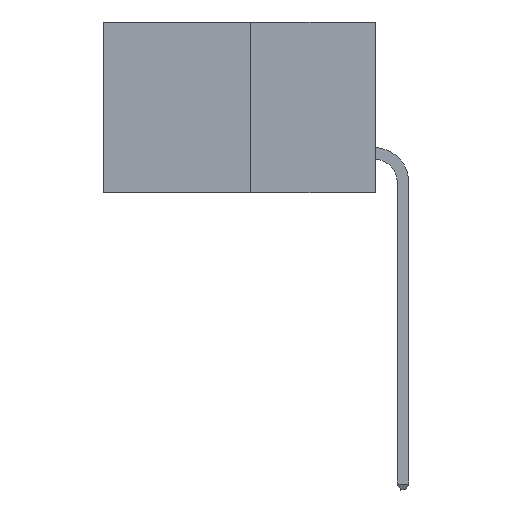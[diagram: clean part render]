
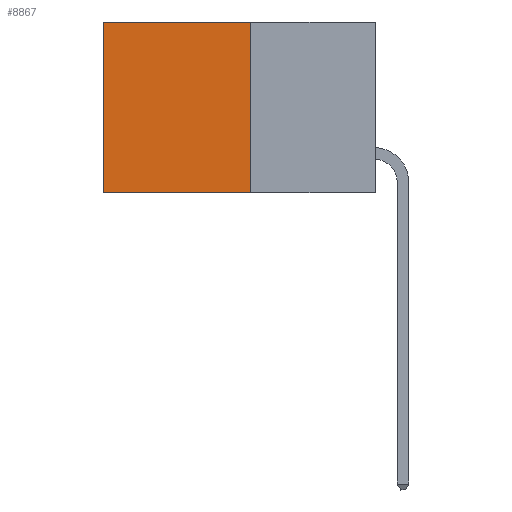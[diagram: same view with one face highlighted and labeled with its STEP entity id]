
A CAD part, left-side view. The second image highlights one B-rep face of the part: STEP entity #8867.
In plain terms, the highlighted planar face has unit normal (-1, 0, 0).
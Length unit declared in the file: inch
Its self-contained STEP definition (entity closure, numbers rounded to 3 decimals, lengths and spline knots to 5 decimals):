
#607 = ORIENTED_EDGE ( 'NONE', *, *, #22650, .F. ) ;
#1175 = CARTESIAN_POINT ( 'NONE',  ( 0.277, 0.27, -0.37 ) ) ;
#1921 = CARTESIAN_POINT ( 'NONE',  ( 0.277, 0.59, -0.37 ) ) ;
#2026 = VECTOR ( 'NONE', #3711, 39.37008 ) ;
#2639 = VECTOR ( 'NONE', #19897, 39.37008 ) ;
#2892 = ORIENTED_EDGE ( 'NONE', *, *, #20036, .T. ) ;
#3202 = DIRECTION ( 'NONE',  ( 0., 0., -1. ) ) ;
#3404 = AXIS2_PLACEMENT_3D ( 'NONE', #17860, #19901, #7704 ) ;
#3520 = PLANE ( 'NONE',  #3404 ) ;
#3711 = DIRECTION ( 'NONE',  ( 0., 1., 0. ) ) ;
#5674 = CARTESIAN_POINT ( 'NONE',  ( 0.277, 0.59, -0.37 ) ) ;
#6026 = DIRECTION ( 'NONE',  ( 0., 0., -1. ) ) ;
#7704 = DIRECTION ( 'NONE',  ( 0., 0., -1. ) ) ;
#7961 = EDGE_CURVE ( 'NONE', #23606, #10825, #8156, .T. ) ;
#8156 = LINE ( 'NONE', #21233, #2639 ) ;
#8506 = VECTOR ( 'NONE', #6026, 39.37008 ) ;
#8867 = ADVANCED_FACE ( 'NONE', ( #13702 ), #3520, .F. ) ;
#9811 = ORIENTED_EDGE ( 'NONE', *, *, #26170, .T. ) ;
#9969 = ORIENTED_EDGE ( 'NONE', *, *, #7961, .F. ) ;
#10407 = VERTEX_POINT ( 'NONE', #12290 ) ;
#10825 = VERTEX_POINT ( 'NONE', #5674 ) ;
#10847 = CARTESIAN_POINT ( 'NONE',  ( 0.277, 0.27, 0. ) ) ;
#11465 = EDGE_LOOP ( 'NONE', ( #2892, #9969, #607, #9811 ) ) ;
#12290 = CARTESIAN_POINT ( 'NONE',  ( 0.277, 0.59, 0. ) ) ;
#13702 = FACE_OUTER_BOUND ( 'NONE', #11465, .T. ) ;
#13933 = LINE ( 'NONE', #1921, #8506 ) ;
#13993 = CARTESIAN_POINT ( 'NONE',  ( 0.277, 0.27, 0. ) ) ;
#17860 = CARTESIAN_POINT ( 'NONE',  ( 0.277, 0.27, -0.37 ) ) ;
#18362 = LINE ( 'NONE', #13993, #2026 ) ;
#19897 = DIRECTION ( 'NONE',  ( 0., 1., 0. ) ) ;
#19901 = DIRECTION ( 'NONE',  ( 1., 0., 0. ) ) ;
#20036 = EDGE_CURVE ( 'NONE', #10407, #10825, #13933, .T. ) ;
#20043 = CARTESIAN_POINT ( 'NONE',  ( 0.277, 0.27, -0.37 ) ) ;
#20389 = VECTOR ( 'NONE', #3202, 39.37008 ) ;
#21233 = CARTESIAN_POINT ( 'NONE',  ( 0.277, 0.27, -0.37 ) ) ;
#21584 = LINE ( 'NONE', #1175, #20389 ) ;
#22650 = EDGE_CURVE ( 'NONE', #24552, #23606, #21584, .T. ) ;
#23606 = VERTEX_POINT ( 'NONE', #20043 ) ;
#24552 = VERTEX_POINT ( 'NONE', #10847 ) ;
#26170 = EDGE_CURVE ( 'NONE', #24552, #10407, #18362, .T. ) ;
